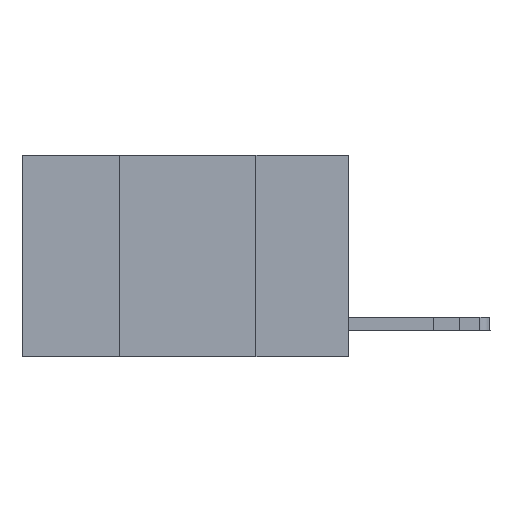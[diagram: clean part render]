
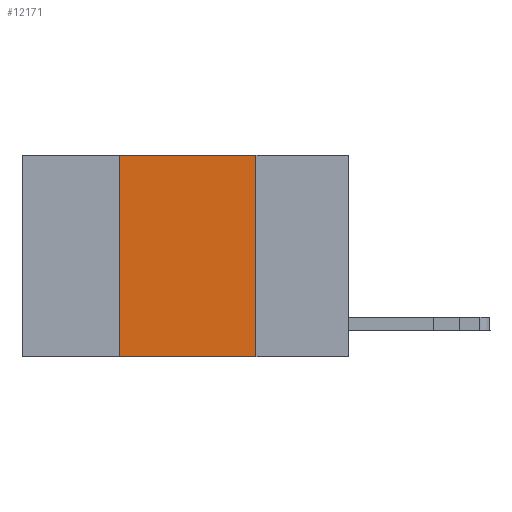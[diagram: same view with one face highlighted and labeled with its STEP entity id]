
A CAD part, left-side view. The second image highlights one B-rep face of the part: STEP entity #12171.
In plain terms, the highlighted planar face has unit normal (-1, 0, 0).
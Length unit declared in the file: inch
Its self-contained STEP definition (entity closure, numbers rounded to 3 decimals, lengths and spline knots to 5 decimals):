
#836 = DIRECTION ( 'NONE',  ( 0., -1., 0. ) ) ;
#1334 = DIRECTION ( 'NONE',  ( 0., 0., 1. ) ) ;
#1412 = EDGE_CURVE ( 'NONE', #1447, #14202, #7854, .T. ) ;
#1447 = VERTEX_POINT ( 'NONE', #6364 ) ;
#1504 = VECTOR ( 'NONE', #836, 39.37008 ) ;
#1927 = ORIENTED_EDGE ( 'NONE', *, *, #10665, .F. ) ;
#3140 = CARTESIAN_POINT ( 'NONE',  ( 0., 0.6, 0. ) ) ;
#4366 = PLANE ( 'NONE',  #6007 ) ;
#4542 = ORIENTED_EDGE ( 'NONE', *, *, #6133, .F. ) ;
#4783 = CARTESIAN_POINT ( 'NONE',  ( 0., 0.17, -0.37 ) ) ;
#5108 = ORIENTED_EDGE ( 'NONE', *, *, #14548, .T. ) ;
#5200 = VECTOR ( 'NONE', #1334, 39.37008 ) ;
#5348 = DIRECTION ( 'NONE',  ( 0., -1., 0. ) ) ;
#6007 = AXIS2_PLACEMENT_3D ( 'NONE', #3140, #6926, #11967 ) ;
#6133 = EDGE_CURVE ( 'NONE', #12298, #11935, #8568, .T. ) ;
#6364 = CARTESIAN_POINT ( 'NONE',  ( 0., 0.42, -0.37 ) ) ;
#6926 = DIRECTION ( 'NONE',  ( 1., 0., 0. ) ) ;
#7263 = DIRECTION ( 'NONE',  ( 0., 0., -1. ) ) ;
#7854 = LINE ( 'NONE', #13890, #5200 ) ;
#7983 = LINE ( 'NONE', #15451, #10777 ) ;
#8332 = LINE ( 'NONE', #12147, #1504 ) ;
#8568 = LINE ( 'NONE', #13704, #11722 ) ;
#10175 = ORIENTED_EDGE ( 'NONE', *, *, #1412, .F. ) ;
#10665 = EDGE_CURVE ( 'NONE', #14202, #12298, #8332, .T. ) ;
#10777 = VECTOR ( 'NONE', #5348, 39.37008 ) ;
#11722 = VECTOR ( 'NONE', #7263, 39.37008 ) ;
#11935 = VERTEX_POINT ( 'NONE', #4783 ) ;
#11967 = DIRECTION ( 'NONE',  ( 0., 0., -1. ) ) ;
#12147 = CARTESIAN_POINT ( 'NONE',  ( 0., 0.6, 0. ) ) ;
#12171 = ADVANCED_FACE ( 'NONE', ( #15714 ), #4366, .F. ) ;
#12212 = CARTESIAN_POINT ( 'NONE',  ( 0., 0.17, 0. ) ) ;
#12298 = VERTEX_POINT ( 'NONE', #12212 ) ;
#12770 = CARTESIAN_POINT ( 'NONE',  ( 0., 0.42, 0. ) ) ;
#13704 = CARTESIAN_POINT ( 'NONE',  ( 0., 0.17, 0. ) ) ;
#13890 = CARTESIAN_POINT ( 'NONE',  ( 0., 0.42, 0. ) ) ;
#14202 = VERTEX_POINT ( 'NONE', #12770 ) ;
#14548 = EDGE_CURVE ( 'NONE', #1447, #11935, #7983, .T. ) ;
#14668 = EDGE_LOOP ( 'NONE', ( #4542, #1927, #10175, #5108 ) ) ;
#15451 = CARTESIAN_POINT ( 'NONE',  ( 0., 0.6, -0.37 ) ) ;
#15714 = FACE_OUTER_BOUND ( 'NONE', #14668, .T. ) ;
